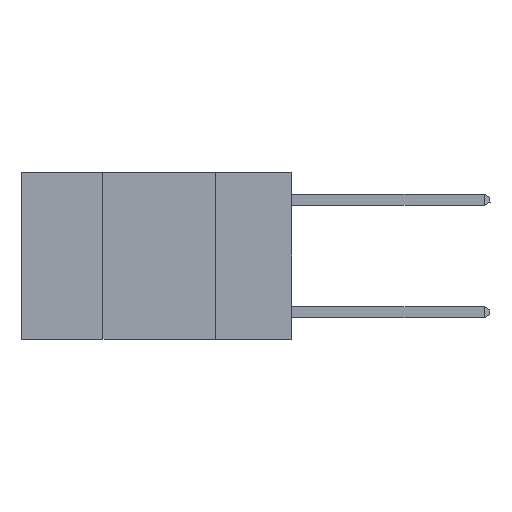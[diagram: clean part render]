
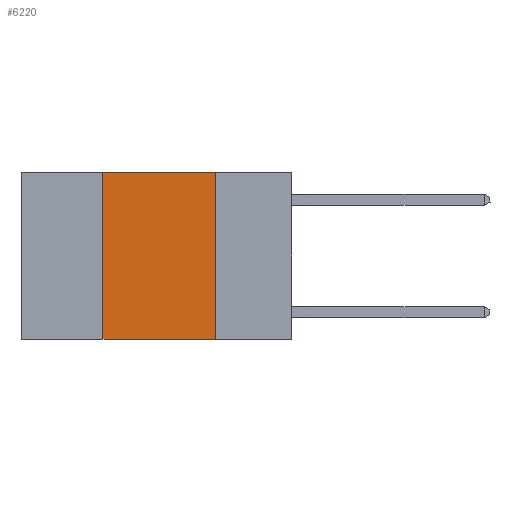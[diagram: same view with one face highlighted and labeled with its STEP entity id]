
A CAD part, left-side view. The second image highlights one B-rep face of the part: STEP entity #6220.
In plain terms, the highlighted planar face has unit normal (-1, 0, 0).
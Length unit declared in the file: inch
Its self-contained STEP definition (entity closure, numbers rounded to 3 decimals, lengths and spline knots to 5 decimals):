
#850 = CARTESIAN_POINT ( 'NONE',  ( 0., 0.42, 0. ) ) ;
#1628 = PLANE ( 'NONE',  #10643 ) ;
#3525 = DIRECTION ( 'NONE',  ( 1., 0., 0. ) ) ;
#3612 = EDGE_CURVE ( 'NONE', #20681, #6691, #21183, .T. ) ;
#4408 = VECTOR ( 'NONE', #5155, 39.37008 ) ;
#5155 = DIRECTION ( 'NONE',  ( 0., -1., 0. ) ) ;
#6220 = ADVANCED_FACE ( 'NONE', ( #11664 ), #1628, .F. ) ;
#6691 = VERTEX_POINT ( 'NONE', #23299 ) ;
#7673 = VECTOR ( 'NONE', #13079, 39.37008 ) ;
#8296 = LINE ( 'NONE', #850, #22378 ) ;
#10492 = ORIENTED_EDGE ( 'NONE', *, *, #16670, .F. ) ;
#10643 = AXIS2_PLACEMENT_3D ( 'NONE', #14814, #3525, #16667 ) ;
#10718 = ORIENTED_EDGE ( 'NONE', *, *, #16621, .F. ) ;
#11192 = CARTESIAN_POINT ( 'NONE',  ( 0., 0.17, 0. ) ) ;
#11664 = FACE_OUTER_BOUND ( 'NONE', #18259, .T. ) ;
#11716 = ORIENTED_EDGE ( 'NONE', *, *, #19122, .F. ) ;
#12960 = VERTEX_POINT ( 'NONE', #16072 ) ;
#13079 = DIRECTION ( 'NONE',  ( 0., 0., -1. ) ) ;
#13801 = LINE ( 'NONE', #18182, #4408 ) ;
#14041 = ORIENTED_EDGE ( 'NONE', *, *, #3612, .T. ) ;
#14218 = CARTESIAN_POINT ( 'NONE',  ( 0., 0.17, 0. ) ) ;
#14814 = CARTESIAN_POINT ( 'NONE',  ( 0., 0.6, 0. ) ) ;
#14921 = CARTESIAN_POINT ( 'NONE',  ( 0., 0.6, -0.37 ) ) ;
#16072 = CARTESIAN_POINT ( 'NONE',  ( 0., 0.42, 0. ) ) ;
#16621 = EDGE_CURVE ( 'NONE', #12960, #19169, #13801, .T. ) ;
#16667 = DIRECTION ( 'NONE',  ( 0., 0., -1. ) ) ;
#16670 = EDGE_CURVE ( 'NONE', #19169, #6691, #17580, .T. ) ;
#17580 = LINE ( 'NONE', #11192, #7673 ) ;
#17684 = DIRECTION ( 'NONE',  ( 0., -1., 0. ) ) ;
#18182 = CARTESIAN_POINT ( 'NONE',  ( 0., 0.6, 0. ) ) ;
#18259 = EDGE_LOOP ( 'NONE', ( #10492, #10718, #11716, #14041 ) ) ;
#19122 = EDGE_CURVE ( 'NONE', #20681, #12960, #8296, .T. ) ;
#19169 = VERTEX_POINT ( 'NONE', #14218 ) ;
#20681 = VERTEX_POINT ( 'NONE', #20895 ) ;
#20895 = CARTESIAN_POINT ( 'NONE',  ( 0., 0.42, -0.37 ) ) ;
#21183 = LINE ( 'NONE', #14921, #21739 ) ;
#21739 = VECTOR ( 'NONE', #17684, 39.37008 ) ;
#22378 = VECTOR ( 'NONE', #23160, 39.37008 ) ;
#23160 = DIRECTION ( 'NONE',  ( 0., 0., 1. ) ) ;
#23299 = CARTESIAN_POINT ( 'NONE',  ( 0., 0.17, -0.37 ) ) ;
